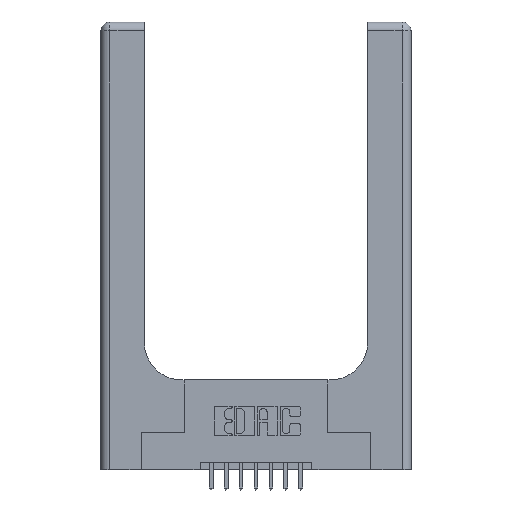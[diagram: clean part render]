
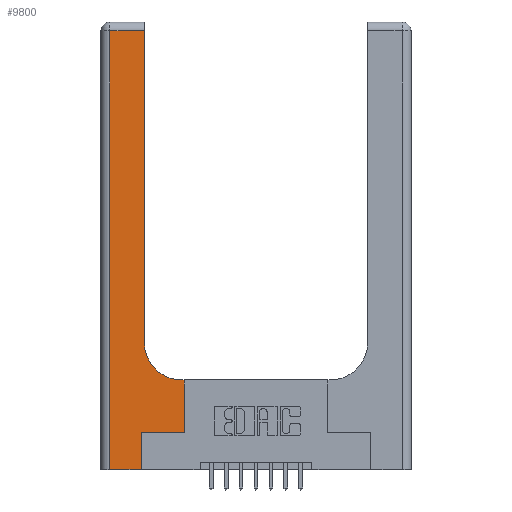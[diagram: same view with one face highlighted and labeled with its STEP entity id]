
A CAD part, top view. The second image highlights one B-rep face of the part: STEP entity #9800.
In plain terms, the highlighted planar face has unit normal (0, 0, 1).
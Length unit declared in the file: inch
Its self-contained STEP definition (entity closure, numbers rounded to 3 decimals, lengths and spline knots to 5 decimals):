
#95 = CARTESIAN_POINT ( 'NONE',  ( 0.2915, 0.85, 0.37 ) ) ;
#155 = EDGE_CURVE ( 'NONE', #2117, #6814, #9730, .T. ) ;
#276 = ORIENTED_EDGE ( 'NONE', *, *, #9265, .T. ) ;
#434 = DIRECTION ( 'NONE',  ( 0., -1., 0. ) ) ;
#485 = CARTESIAN_POINT ( 'NONE',  ( 0.06, 3., 0.37 ) ) ;
#578 = CARTESIAN_POINT ( 'NONE',  ( 0.269, 0., 0.37 ) ) ;
#1273 = LINE ( 'NONE', #485, #13590 ) ;
#1386 = LINE ( 'NONE', #578, #13705 ) ;
#1495 = VECTOR ( 'NONE', #12256, 39.37008 ) ;
#1811 = CARTESIAN_POINT ( 'NONE',  ( 0.5585, 0.6, 0.37 ) ) ;
#2000 = EDGE_CURVE ( 'NONE', #12690, #13473, #7885, .T. ) ;
#2025 = CARTESIAN_POINT ( 'NONE',  ( 0., 3., 0.37 ) ) ;
#2073 = DIRECTION ( 'NONE',  ( 0., 0., -1. ) ) ;
#2117 = VERTEX_POINT ( 'NONE', #6714 ) ;
#2252 = DIRECTION ( 'NONE',  ( 0., 1., 0. ) ) ;
#2678 = EDGE_CURVE ( 'NONE', #13577, #11618, #15054, .T. ) ;
#2745 = CARTESIAN_POINT ( 'NONE',  ( 0.5585, 0.25, 0.37 ) ) ;
#2781 = EDGE_CURVE ( 'NONE', #11618, #7253, #13600, .T. ) ;
#3271 = EDGE_CURVE ( 'NONE', #6814, #12690, #1273, .T. ) ;
#3861 = DIRECTION ( 'NONE',  ( 1., 0., 0. ) ) ;
#4098 = VECTOR ( 'NONE', #2252, 39.37008 ) ;
#4156 = CARTESIAN_POINT ( 'NONE',  ( 0.2915, 3., 0.37 ) ) ;
#4192 = CARTESIAN_POINT ( 'NONE',  ( 0.06, 2.94, 0.37 ) ) ;
#4595 = VECTOR ( 'NONE', #7502, 39.37008 ) ;
#4686 = CARTESIAN_POINT ( 'NONE',  ( 0.269, 0.25, 0.37 ) ) ;
#4980 = ORIENTED_EDGE ( 'NONE', *, *, #6297, .T. ) ;
#5268 = CARTESIAN_POINT ( 'NONE',  ( 0.269, 0., 0.37 ) ) ;
#5601 = VECTOR ( 'NONE', #3861, 39.37008 ) ;
#5679 = CIRCLE ( 'NONE', #8410, 0.25 ) ;
#5765 = DIRECTION ( 'NONE',  ( 0., 0., -1. ) ) ;
#6290 = CARTESIAN_POINT ( 'NONE',  ( 0.2915, 0.6, 0.37 ) ) ;
#6297 = EDGE_CURVE ( 'NONE', #12117, #6546, #5679, .T. ) ;
#6546 = VERTEX_POINT ( 'NONE', #95 ) ;
#6652 = ORIENTED_EDGE ( 'NONE', *, *, #2678, .T. ) ;
#6714 = CARTESIAN_POINT ( 'NONE',  ( 0.2915, 2.94, 0.37 ) ) ;
#6814 = VERTEX_POINT ( 'NONE', #4192 ) ;
#6860 = CARTESIAN_POINT ( 'NONE',  ( 0.06, 0., 0.37 ) ) ;
#7207 = FACE_OUTER_BOUND ( 'NONE', #8274, .T. ) ;
#7253 = VERTEX_POINT ( 'NONE', #1811 ) ;
#7277 = DIRECTION ( 'NONE',  ( -1., 0., 0. ) ) ;
#7407 = ORIENTED_EDGE ( 'NONE', *, *, #2781, .T. ) ;
#7435 = CARTESIAN_POINT ( 'NONE',  ( 0., 2.94, 0.37 ) ) ;
#7502 = DIRECTION ( 'NONE',  ( -1., 0., 0. ) ) ;
#7885 = LINE ( 'NONE', #9131, #1495 ) ;
#8038 = AXIS2_PLACEMENT_3D ( 'NONE', #2025, #2073, #10472 ) ;
#8274 = EDGE_LOOP ( 'NONE', ( #14261, #14619, #12243, #12622, #276, #6652, #7407, #14083, #4980 ) ) ;
#8410 = AXIS2_PLACEMENT_3D ( 'NONE', #12923, #5765, #14088 ) ;
#9019 = VECTOR ( 'NONE', #7277, 39.37008 ) ;
#9131 = CARTESIAN_POINT ( 'NONE',  ( 0., 0., 0.37 ) ) ;
#9265 = EDGE_CURVE ( 'NONE', #13473, #13577, #1386, .T. ) ;
#9279 = PLANE ( 'NONE',  #8038 ) ;
#9341 = CARTESIAN_POINT ( 'NONE',  ( 0.5415, 0.6, 0.37 ) ) ;
#9479 = EDGE_CURVE ( 'NONE', #7253, #12117, #13885, .T. ) ;
#9730 = LINE ( 'NONE', #7435, #9019 ) ;
#9800 = ADVANCED_FACE ( 'NONE', ( #7207 ), #9279, .F. ) ;
#10472 = DIRECTION ( 'NONE',  ( -1., 0., 0. ) ) ;
#10872 = EDGE_CURVE ( 'NONE', #6546, #2117, #14401, .T. ) ;
#11353 = DIRECTION ( 'NONE',  ( 0., 1., 0. ) ) ;
#11618 = VERTEX_POINT ( 'NONE', #15076 ) ;
#12117 = VERTEX_POINT ( 'NONE', #9341 ) ;
#12243 = ORIENTED_EDGE ( 'NONE', *, *, #3271, .T. ) ;
#12256 = DIRECTION ( 'NONE',  ( 1., 0., 0. ) ) ;
#12622 = ORIENTED_EDGE ( 'NONE', *, *, #2000, .T. ) ;
#12690 = VERTEX_POINT ( 'NONE', #6860 ) ;
#12923 = CARTESIAN_POINT ( 'NONE',  ( 0.5415, 0.85, 0.37 ) ) ;
#13473 = VERTEX_POINT ( 'NONE', #5268 ) ;
#13577 = VERTEX_POINT ( 'NONE', #14953 ) ;
#13590 = VECTOR ( 'NONE', #434, 39.37008 ) ;
#13600 = LINE ( 'NONE', #2745, #4098 ) ;
#13688 = DIRECTION ( 'NONE',  ( 0., 1., 0. ) ) ;
#13705 = VECTOR ( 'NONE', #11353, 39.37008 ) ;
#13885 = LINE ( 'NONE', #6290, #4595 ) ;
#14042 = VECTOR ( 'NONE', #13688, 39.37008 ) ;
#14083 = ORIENTED_EDGE ( 'NONE', *, *, #9479, .T. ) ;
#14088 = DIRECTION ( 'NONE',  ( 1., 0., 0. ) ) ;
#14261 = ORIENTED_EDGE ( 'NONE', *, *, #10872, .T. ) ;
#14401 = LINE ( 'NONE', #4156, #14042 ) ;
#14619 = ORIENTED_EDGE ( 'NONE', *, *, #155, .T. ) ;
#14953 = CARTESIAN_POINT ( 'NONE',  ( 0.269, 0.25, 0.37 ) ) ;
#15054 = LINE ( 'NONE', #4686, #5601 ) ;
#15076 = CARTESIAN_POINT ( 'NONE',  ( 0.5585, 0.25, 0.37 ) ) ;
